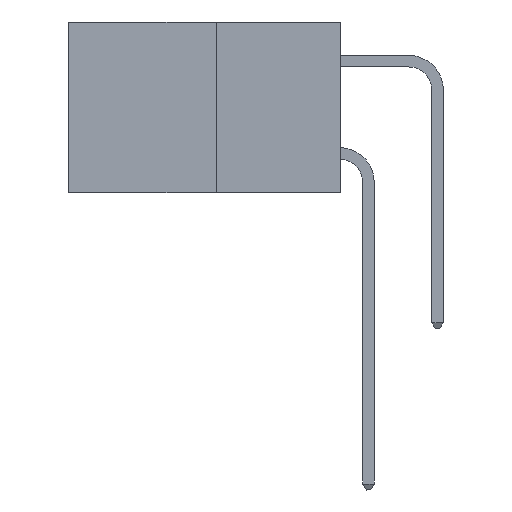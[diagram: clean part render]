
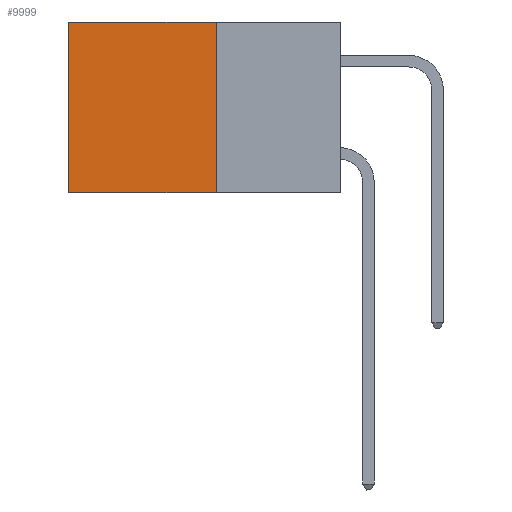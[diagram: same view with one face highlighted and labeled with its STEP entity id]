
A CAD part, left-side view. The second image highlights one B-rep face of the part: STEP entity #9999.
In plain terms, the highlighted planar face has unit normal (-1, 0, 0).
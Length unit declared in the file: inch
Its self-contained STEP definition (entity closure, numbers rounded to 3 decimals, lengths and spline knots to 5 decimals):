
#367 = VERTEX_POINT ( 'NONE', #13962 ) ;
#1169 = CARTESIAN_POINT ( 'NONE',  ( 0.277, 0.59, 0. ) ) ;
#1984 = EDGE_CURVE ( 'NONE', #367, #18137, #20451, .T. ) ;
#2342 = EDGE_CURVE ( 'NONE', #367, #9208, #17190, .T. ) ;
#2978 = VECTOR ( 'NONE', #13115, 39.37008 ) ;
#5526 = CARTESIAN_POINT ( 'NONE',  ( 0.277, 0.59, -0.37 ) ) ;
#5895 = ORIENTED_EDGE ( 'NONE', *, *, #2342, .F. ) ;
#6184 = VERTEX_POINT ( 'NONE', #5526 ) ;
#7777 = EDGE_LOOP ( 'NONE', ( #13676, #14911, #5895, #24036 ) ) ;
#9208 = VERTEX_POINT ( 'NONE', #13868 ) ;
#9999 = ADVANCED_FACE ( 'NONE', ( #18891 ), #14495, .F. ) ;
#10137 = VECTOR ( 'NONE', #22927, 39.37008 ) ;
#11012 = EDGE_CURVE ( 'NONE', #9208, #6184, #15180, .T. ) ;
#12650 = DIRECTION ( 'NONE',  ( 0., 0., -1. ) ) ;
#12801 = CARTESIAN_POINT ( 'NONE',  ( 0.277, 0.27, 0. ) ) ;
#13115 = DIRECTION ( 'NONE',  ( 0., 0., -1. ) ) ;
#13447 = CARTESIAN_POINT ( 'NONE',  ( 0.277, 0.27, -0.37 ) ) ;
#13676 = ORIENTED_EDGE ( 'NONE', *, *, #24474, .T. ) ;
#13868 = CARTESIAN_POINT ( 'NONE',  ( 0.277, 0.27, -0.37 ) ) ;
#13962 = CARTESIAN_POINT ( 'NONE',  ( 0.277, 0.27, 0. ) ) ;
#14304 = VECTOR ( 'NONE', #18986, 39.37008 ) ;
#14495 = PLANE ( 'NONE',  #20325 ) ;
#14911 = ORIENTED_EDGE ( 'NONE', *, *, #11012, .F. ) ;
#15180 = LINE ( 'NONE', #13447, #10137 ) ;
#16580 = VECTOR ( 'NONE', #19996, 39.37008 ) ;
#17190 = LINE ( 'NONE', #20527, #16580 ) ;
#18137 = VERTEX_POINT ( 'NONE', #1169 ) ;
#18891 = FACE_OUTER_BOUND ( 'NONE', #7777, .T. ) ;
#18986 = DIRECTION ( 'NONE',  ( 0., 1., 0. ) ) ;
#19996 = DIRECTION ( 'NONE',  ( 0., 0., -1. ) ) ;
#20230 = CARTESIAN_POINT ( 'NONE',  ( 0.277, 0.27, -0.37 ) ) ;
#20325 = AXIS2_PLACEMENT_3D ( 'NONE', #20230, #23937, #12650 ) ;
#20451 = LINE ( 'NONE', #12801, #14304 ) ;
#20527 = CARTESIAN_POINT ( 'NONE',  ( 0.277, 0.27, -0.37 ) ) ;
#22756 = LINE ( 'NONE', #24367, #2978 ) ;
#22927 = DIRECTION ( 'NONE',  ( 0., 1., 0. ) ) ;
#23937 = DIRECTION ( 'NONE',  ( 1., 0., 0. ) ) ;
#24036 = ORIENTED_EDGE ( 'NONE', *, *, #1984, .T. ) ;
#24367 = CARTESIAN_POINT ( 'NONE',  ( 0.277, 0.59, -0.37 ) ) ;
#24474 = EDGE_CURVE ( 'NONE', #18137, #6184, #22756, .T. ) ;
